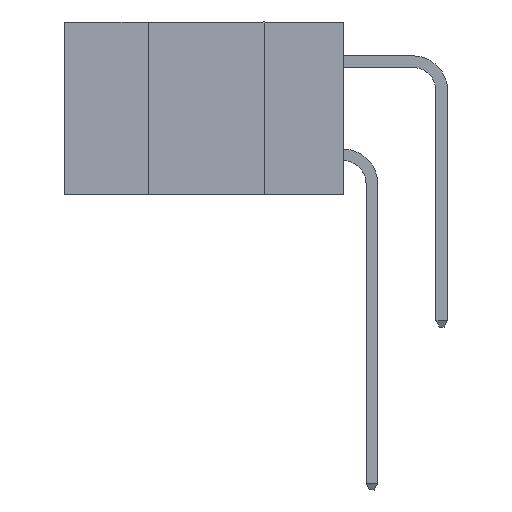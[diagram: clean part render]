
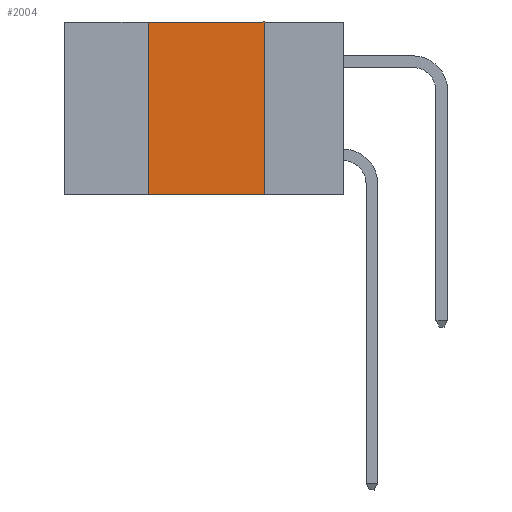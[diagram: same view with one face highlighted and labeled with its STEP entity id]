
A CAD part, left-side view. The second image highlights one B-rep face of the part: STEP entity #2004.
In plain terms, the highlighted planar face has unit normal (-1, 0, 0).
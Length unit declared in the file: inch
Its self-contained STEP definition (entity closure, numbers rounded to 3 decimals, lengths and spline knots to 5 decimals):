
#442 = EDGE_CURVE ( 'NONE', #13252, #1415, #1961, .T. ) ;
#1286 = DIRECTION ( 'NONE',  ( 0., 0., -1. ) ) ;
#1415 = VERTEX_POINT ( 'NONE', #2331 ) ;
#1961 = LINE ( 'NONE', #18140, #2555 ) ;
#2004 = ADVANCED_FACE ( 'NONE', ( #18702 ), #5596, .F. ) ;
#2228 = CARTESIAN_POINT ( 'NONE',  ( 0., 0.17, 0. ) ) ;
#2331 = CARTESIAN_POINT ( 'NONE',  ( 0., 0.17, -0.37 ) ) ;
#2555 = VECTOR ( 'NONE', #21005, 39.37008 ) ;
#2743 = VECTOR ( 'NONE', #9475, 39.37008 ) ;
#3028 = EDGE_CURVE ( 'NONE', #16709, #1415, #3326, .T. ) ;
#3326 = LINE ( 'NONE', #4814, #2743 ) ;
#3649 = CARTESIAN_POINT ( 'NONE',  ( 0., 0.6, 0. ) ) ;
#4363 = DIRECTION ( 'NONE',  ( 0., 0., 1. ) ) ;
#4814 = CARTESIAN_POINT ( 'NONE',  ( 0., 0.17, -0.37 ) ) ;
#5457 = ORIENTED_EDGE ( 'NONE', *, *, #10472, .F. ) ;
#5498 = VECTOR ( 'NONE', #4363, 39.37008 ) ;
#5596 = PLANE ( 'NONE',  #19756 ) ;
#5936 = DIRECTION ( 'NONE',  ( 1., 0., 0. ) ) ;
#7916 = CARTESIAN_POINT ( 'NONE',  ( 0., 0.42, 0. ) ) ;
#8204 = VECTOR ( 'NONE', #15477, 39.37008 ) ;
#8460 = EDGE_CURVE ( 'NONE', #11515, #16709, #18026, .T. ) ;
#9215 = ORIENTED_EDGE ( 'NONE', *, *, #8460, .F. ) ;
#9475 = DIRECTION ( 'NONE',  ( 0., 0., -1. ) ) ;
#9885 = CARTESIAN_POINT ( 'NONE',  ( 0., 0.42, -0.37 ) ) ;
#10103 = ORIENTED_EDGE ( 'NONE', *, *, #3028, .F. ) ;
#10472 = EDGE_CURVE ( 'NONE', #13252, #11515, #11026, .T. ) ;
#11026 = LINE ( 'NONE', #9885, #5498 ) ;
#11515 = VERTEX_POINT ( 'NONE', #7916 ) ;
#13252 = VERTEX_POINT ( 'NONE', #22096 ) ;
#13624 = CARTESIAN_POINT ( 'NONE',  ( 0., 0.6, 0. ) ) ;
#15477 = DIRECTION ( 'NONE',  ( 0., -1., 0. ) ) ;
#16709 = VERTEX_POINT ( 'NONE', #2228 ) ;
#17252 = EDGE_LOOP ( 'NONE', ( #10103, #9215, #5457, #22809 ) ) ;
#18026 = LINE ( 'NONE', #13624, #8204 ) ;
#18140 = CARTESIAN_POINT ( 'NONE',  ( 0., 0.6, -0.37 ) ) ;
#18702 = FACE_OUTER_BOUND ( 'NONE', #17252, .T. ) ;
#19756 = AXIS2_PLACEMENT_3D ( 'NONE', #3649, #5936, #1286 ) ;
#21005 = DIRECTION ( 'NONE',  ( 0., -1., 0. ) ) ;
#22096 = CARTESIAN_POINT ( 'NONE',  ( 0., 0.42, -0.37 ) ) ;
#22809 = ORIENTED_EDGE ( 'NONE', *, *, #442, .T. ) ;
